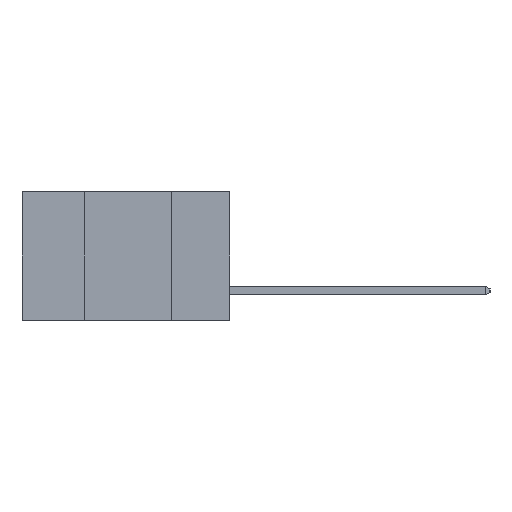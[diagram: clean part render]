
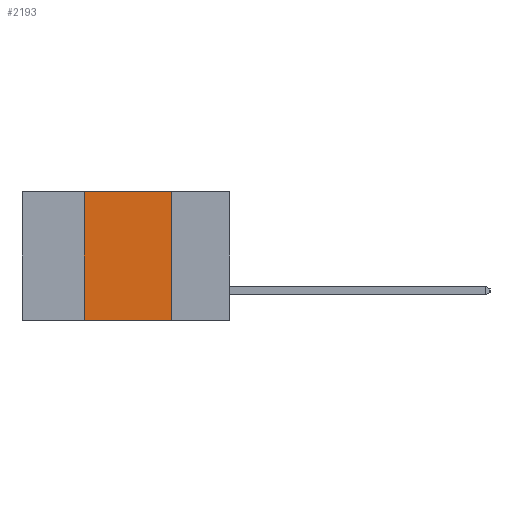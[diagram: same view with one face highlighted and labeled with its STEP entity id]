
A CAD part, left-side view. The second image highlights one B-rep face of the part: STEP entity #2193.
In plain terms, the highlighted planar face has unit normal (-1, 0, 0).
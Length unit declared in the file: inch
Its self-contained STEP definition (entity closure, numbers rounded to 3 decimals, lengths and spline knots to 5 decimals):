
#426 = FACE_OUTER_BOUND ( 'NONE', #863, .T. ) ;
#863 = EDGE_LOOP ( 'NONE', ( #8849, #5507, #17022, #2504 ) ) ;
#1748 = VECTOR ( 'NONE', #7916, 39.37008 ) ;
#2193 = ADVANCED_FACE ( 'NONE', ( #426 ), #13232, .F. ) ;
#2286 = DIRECTION ( 'NONE',  ( 0., 0., -1. ) ) ;
#2504 = ORIENTED_EDGE ( 'NONE', *, *, #2914, .T. ) ;
#2688 = VECTOR ( 'NONE', #18557, 39.37008 ) ;
#2906 = LINE ( 'NONE', #11983, #6607 ) ;
#2914 = EDGE_CURVE ( 'NONE', #7596, #9113, #2906, .T. ) ;
#3962 = EDGE_CURVE ( 'NONE', #7596, #10492, #11062, .T. ) ;
#4061 = CARTESIAN_POINT ( 'NONE',  ( 0., 0.42, 0. ) ) ;
#5114 = DIRECTION ( 'NONE',  ( 1., 0., 0. ) ) ;
#5507 = ORIENTED_EDGE ( 'NONE', *, *, #7163, .F. ) ;
#6607 = VECTOR ( 'NONE', #12106, 39.37008 ) ;
#6904 = CARTESIAN_POINT ( 'NONE',  ( 0., 0.17, -0.37 ) ) ;
#7163 = EDGE_CURVE ( 'NONE', #10492, #14600, #13600, .T. ) ;
#7596 = VERTEX_POINT ( 'NONE', #7690 ) ;
#7690 = CARTESIAN_POINT ( 'NONE',  ( 0., 0.42, -0.37 ) ) ;
#7916 = DIRECTION ( 'NONE',  ( 0., 0., -1. ) ) ;
#8188 = EDGE_CURVE ( 'NONE', #14600, #9113, #14258, .T. ) ;
#8779 = CARTESIAN_POINT ( 'NONE',  ( 0., 0.17, -0.37 ) ) ;
#8849 = ORIENTED_EDGE ( 'NONE', *, *, #8188, .F. ) ;
#8935 = VECTOR ( 'NONE', #14565, 39.37008 ) ;
#9113 = VERTEX_POINT ( 'NONE', #6904 ) ;
#10492 = VERTEX_POINT ( 'NONE', #4061 ) ;
#11062 = LINE ( 'NONE', #18708, #2688 ) ;
#11911 = CARTESIAN_POINT ( 'NONE',  ( 0., 0.6, 0. ) ) ;
#11983 = CARTESIAN_POINT ( 'NONE',  ( 0., 0.6, -0.37 ) ) ;
#12106 = DIRECTION ( 'NONE',  ( 0., -1., 0. ) ) ;
#13232 = PLANE ( 'NONE',  #18640 ) ;
#13600 = LINE ( 'NONE', #14644, #8935 ) ;
#14258 = LINE ( 'NONE', #8779, #1748 ) ;
#14565 = DIRECTION ( 'NONE',  ( 0., -1., 0. ) ) ;
#14600 = VERTEX_POINT ( 'NONE', #18044 ) ;
#14644 = CARTESIAN_POINT ( 'NONE',  ( 0., 0.6, 0. ) ) ;
#17022 = ORIENTED_EDGE ( 'NONE', *, *, #3962, .F. ) ;
#18044 = CARTESIAN_POINT ( 'NONE',  ( 0., 0.17, 0. ) ) ;
#18557 = DIRECTION ( 'NONE',  ( 0., 0., 1. ) ) ;
#18640 = AXIS2_PLACEMENT_3D ( 'NONE', #11911, #5114, #2286 ) ;
#18708 = CARTESIAN_POINT ( 'NONE',  ( 0., 0.42, -0.37 ) ) ;
